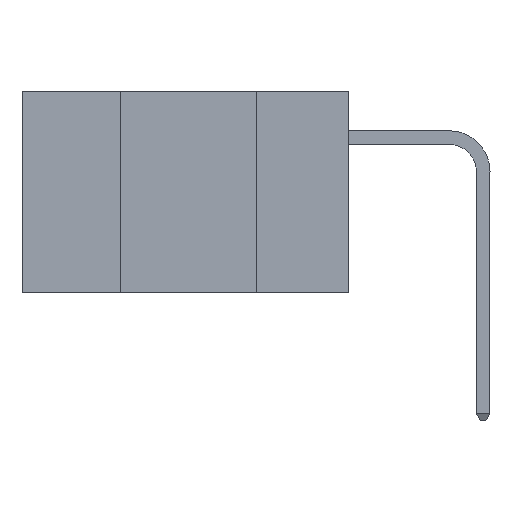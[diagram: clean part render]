
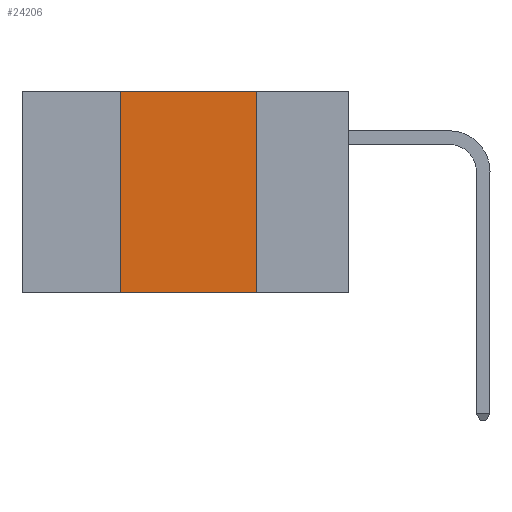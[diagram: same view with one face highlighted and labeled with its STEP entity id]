
A CAD part, left-side view. The second image highlights one B-rep face of the part: STEP entity #24206.
In plain terms, the highlighted planar face has unit normal (-1, 0, 0).
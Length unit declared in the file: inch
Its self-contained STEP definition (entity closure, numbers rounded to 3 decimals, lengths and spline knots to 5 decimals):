
#598 = CARTESIAN_POINT ( 'NONE',  ( 0., 0.6, 0. ) ) ;
#916 = CARTESIAN_POINT ( 'NONE',  ( 0., 0.17, -0.37 ) ) ;
#1524 = CARTESIAN_POINT ( 'NONE',  ( 0., 0.17, 0. ) ) ;
#2300 = LINE ( 'NONE', #11938, #23665 ) ;
#2597 = LINE ( 'NONE', #22082, #7497 ) ;
#4796 = EDGE_CURVE ( 'NONE', #19408, #12662, #2300, .T. ) ;
#6199 = EDGE_CURVE ( 'NONE', #12662, #7496, #16564, .T. ) ;
#6507 = CARTESIAN_POINT ( 'NONE',  ( 0., 0.17, 0. ) ) ;
#6651 = VECTOR ( 'NONE', #8956, 39.37008 ) ;
#7285 = ORIENTED_EDGE ( 'NONE', *, *, #4796, .F. ) ;
#7496 = VERTEX_POINT ( 'NONE', #916 ) ;
#7497 = VECTOR ( 'NONE', #17950, 39.37008 ) ;
#7615 = VERTEX_POINT ( 'NONE', #24107 ) ;
#7736 = EDGE_LOOP ( 'NONE', ( #17674, #7285, #13477, #24395 ) ) ;
#8956 = DIRECTION ( 'NONE',  ( 0., -1., 0. ) ) ;
#9007 = PLANE ( 'NONE',  #15414 ) ;
#11113 = DIRECTION ( 'NONE',  ( 1., 0., 0. ) ) ;
#11938 = CARTESIAN_POINT ( 'NONE',  ( 0., 0.6, 0. ) ) ;
#12465 = CARTESIAN_POINT ( 'NONE',  ( 0., 0.42, 0. ) ) ;
#12662 = VERTEX_POINT ( 'NONE', #1524 ) ;
#12839 = LINE ( 'NONE', #23408, #6651 ) ;
#13477 = ORIENTED_EDGE ( 'NONE', *, *, #16315, .F. ) ;
#14045 = DIRECTION ( 'NONE',  ( 0., -1., 0. ) ) ;
#14803 = DIRECTION ( 'NONE',  ( 0., 0., -1. ) ) ;
#15414 = AXIS2_PLACEMENT_3D ( 'NONE', #598, #11113, #25495 ) ;
#16315 = EDGE_CURVE ( 'NONE', #7615, #19408, #2597, .T. ) ;
#16564 = LINE ( 'NONE', #6507, #21393 ) ;
#16608 = FACE_OUTER_BOUND ( 'NONE', #7736, .T. ) ;
#17674 = ORIENTED_EDGE ( 'NONE', *, *, #6199, .F. ) ;
#17950 = DIRECTION ( 'NONE',  ( 0., 0., 1. ) ) ;
#19408 = VERTEX_POINT ( 'NONE', #12465 ) ;
#21393 = VECTOR ( 'NONE', #14803, 39.37008 ) ;
#21822 = EDGE_CURVE ( 'NONE', #7615, #7496, #12839, .T. ) ;
#22082 = CARTESIAN_POINT ( 'NONE',  ( 0., 0.42, 0. ) ) ;
#23408 = CARTESIAN_POINT ( 'NONE',  ( 0., 0.6, -0.37 ) ) ;
#23665 = VECTOR ( 'NONE', #14045, 39.37008 ) ;
#24107 = CARTESIAN_POINT ( 'NONE',  ( 0., 0.42, -0.37 ) ) ;
#24206 = ADVANCED_FACE ( 'NONE', ( #16608 ), #9007, .F. ) ;
#24395 = ORIENTED_EDGE ( 'NONE', *, *, #21822, .T. ) ;
#25495 = DIRECTION ( 'NONE',  ( 0., 0., -1. ) ) ;
